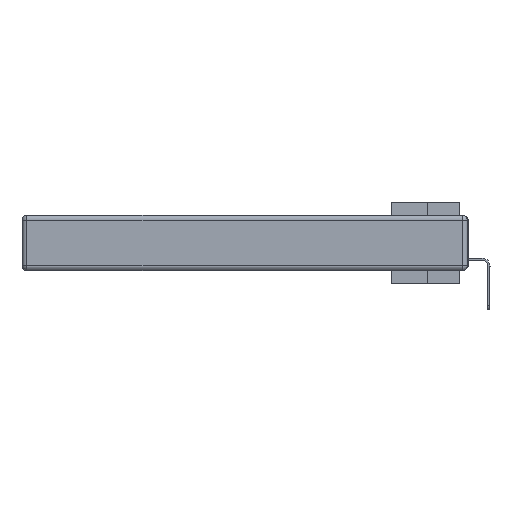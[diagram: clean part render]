
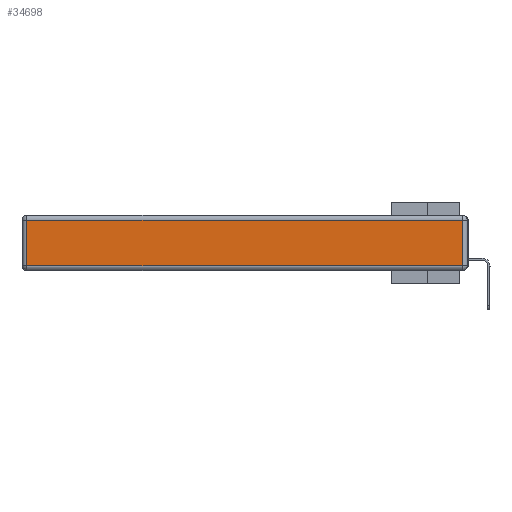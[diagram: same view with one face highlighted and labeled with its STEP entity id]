
A CAD part, left-side view. The second image highlights one B-rep face of the part: STEP entity #34698.
In plain terms, the highlighted planar face has unit normal (-1, 0, 0).
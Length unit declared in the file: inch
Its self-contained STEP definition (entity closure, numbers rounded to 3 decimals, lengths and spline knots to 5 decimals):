
#964 = PLANE ( 'NONE',  #15519 ) ;
#1020 = EDGE_CURVE ( 'NONE', #8362, #32000, #4761, .T. ) ;
#1277 = EDGE_LOOP ( 'NONE', ( #17964, #21833, #21949, #21915 ) ) ;
#2349 = FACE_OUTER_BOUND ( 'NONE', #1277, .T. ) ;
#2467 = VECTOR ( 'NONE', #37802, 39.37008 ) ;
#3956 = DIRECTION ( 'NONE',  ( 0., 0., 1. ) ) ;
#4177 = EDGE_CURVE ( 'NONE', #6377, #11895, #6349, .T. ) ;
#4761 = LINE ( 'NONE', #22895, #10300 ) ;
#5342 = DIRECTION ( 'NONE',  ( 0., 1., 0. ) ) ;
#6349 = LINE ( 'NONE', #17002, #7288 ) ;
#6377 = VERTEX_POINT ( 'NONE', #27424 ) ;
#7288 = VECTOR ( 'NONE', #5342, 39.37008 ) ;
#7703 = CARTESIAN_POINT ( 'NONE',  ( 0., 0.03, -0.313 ) ) ;
#8362 = VERTEX_POINT ( 'NONE', #33910 ) ;
#10300 = VECTOR ( 'NONE', #28692, 39.37008 ) ;
#11895 = VERTEX_POINT ( 'NONE', #18634 ) ;
#12510 = LINE ( 'NONE', #14157, #18000 ) ;
#14157 = CARTESIAN_POINT ( 'NONE',  ( 0., 0.03, -0.343 ) ) ;
#15519 = AXIS2_PLACEMENT_3D ( 'NONE', #33154, #18471, #3956 ) ;
#17002 = CARTESIAN_POINT ( 'NONE',  ( 0., 2.75, -0.03 ) ) ;
#17109 = DIRECTION ( 'NONE',  ( 0., 0., 1. ) ) ;
#17964 = ORIENTED_EDGE ( 'NONE', *, *, #1020, .T. ) ;
#18000 = VECTOR ( 'NONE', #17109, 39.37008 ) ;
#18471 = DIRECTION ( 'NONE',  ( -1., 0., 0. ) ) ;
#18634 = CARTESIAN_POINT ( 'NONE',  ( 0., 2.72, -0.03 ) ) ;
#20390 = LINE ( 'NONE', #37288, #2467 ) ;
#21833 = ORIENTED_EDGE ( 'NONE', *, *, #37988, .T. ) ;
#21915 = ORIENTED_EDGE ( 'NONE', *, *, #33384, .T. ) ;
#21949 = ORIENTED_EDGE ( 'NONE', *, *, #4177, .T. ) ;
#22895 = CARTESIAN_POINT ( 'NONE',  ( 0., 0., -0.313 ) ) ;
#27424 = CARTESIAN_POINT ( 'NONE',  ( 0., 0.03, -0.03 ) ) ;
#28692 = DIRECTION ( 'NONE',  ( 0., -1., 0. ) ) ;
#32000 = VERTEX_POINT ( 'NONE', #7703 ) ;
#33154 = CARTESIAN_POINT ( 'NONE',  ( 0., 0., -0.343 ) ) ;
#33384 = EDGE_CURVE ( 'NONE', #11895, #8362, #20390, .T. ) ;
#33910 = CARTESIAN_POINT ( 'NONE',  ( 0., 2.72, -0.313 ) ) ;
#34698 = ADVANCED_FACE ( 'NONE', ( #2349 ), #964, .T. ) ;
#37288 = CARTESIAN_POINT ( 'NONE',  ( 0., 2.72, -0.343 ) ) ;
#37802 = DIRECTION ( 'NONE',  ( 0., 0., -1. ) ) ;
#37988 = EDGE_CURVE ( 'NONE', #32000, #6377, #12510, .T. ) ;
